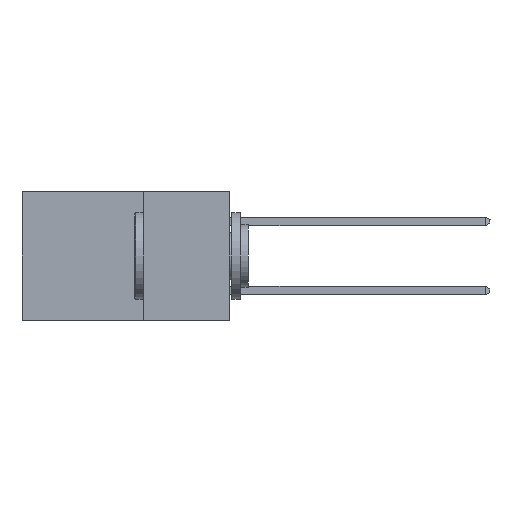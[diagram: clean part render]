
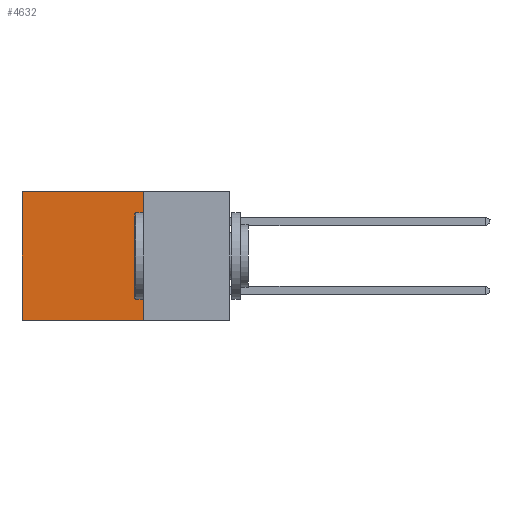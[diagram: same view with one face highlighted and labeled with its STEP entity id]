
A CAD part, left-side view. The second image highlights one B-rep face of the part: STEP entity #4632.
In plain terms, the highlighted planar face has unit normal (-1, 0, 0).
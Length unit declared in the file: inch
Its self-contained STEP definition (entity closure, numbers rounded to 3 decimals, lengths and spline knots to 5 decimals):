
#165 = LINE ( 'NONE', #15744, #16355 ) ;
#769 = EDGE_CURVE ( 'NONE', #20428, #2796, #25912, .T. ) ;
#1388 = DIRECTION ( 'NONE',  ( 0., 0., -1. ) ) ;
#1730 = CARTESIAN_POINT ( 'NONE',  ( 0.298, 0.25, -0.37 ) ) ;
#2405 = DIRECTION ( 'NONE',  ( 0., 1., 0. ) ) ;
#2796 = VERTEX_POINT ( 'NONE', #20936 ) ;
#2900 = VECTOR ( 'NONE', #12399, 39.37008 ) ;
#3042 = FACE_OUTER_BOUND ( 'NONE', #8528, .T. ) ;
#3528 = LINE ( 'NONE', #8315, #2900 ) ;
#4632 = ADVANCED_FACE ( 'NONE', ( #3042 ), #19591, .F. ) ;
#4899 = ORIENTED_EDGE ( 'NONE', *, *, #10779, .T. ) ;
#6405 = CARTESIAN_POINT ( 'NONE',  ( 0.298, 0.25, 0. ) ) ;
#6720 = VECTOR ( 'NONE', #2405, 39.37008 ) ;
#6806 = CARTESIAN_POINT ( 'NONE',  ( 0.298, 0.25, 0. ) ) ;
#6865 = DIRECTION ( 'NONE',  ( 1., 0., 0. ) ) ;
#7548 = DIRECTION ( 'NONE',  ( 0., 0., -1. ) ) ;
#8315 = CARTESIAN_POINT ( 'NONE',  ( 0.298, 0.25, -0.37 ) ) ;
#8528 = EDGE_LOOP ( 'NONE', ( #22389, #21306, #22111, #4899 ) ) ;
#10779 = EDGE_CURVE ( 'NONE', #15896, #20428, #12158, .T. ) ;
#12158 = LINE ( 'NONE', #6405, #6720 ) ;
#12399 = DIRECTION ( 'NONE',  ( 0., 1., 0. ) ) ;
#14059 = EDGE_CURVE ( 'NONE', #22234, #2796, #3528, .T. ) ;
#15744 = CARTESIAN_POINT ( 'NONE',  ( 0.298, 0.25, 0. ) ) ;
#15751 = CARTESIAN_POINT ( 'NONE',  ( 0.298, 0.6, 0. ) ) ;
#15896 = VERTEX_POINT ( 'NONE', #17859 ) ;
#16355 = VECTOR ( 'NONE', #7548, 39.37008 ) ;
#17859 = CARTESIAN_POINT ( 'NONE',  ( 0.298, 0.25, 0. ) ) ;
#19074 = EDGE_CURVE ( 'NONE', #15896, #22234, #165, .T. ) ;
#19461 = VECTOR ( 'NONE', #1388, 39.37008 ) ;
#19591 = PLANE ( 'NONE',  #25476 ) ;
#19594 = DIRECTION ( 'NONE',  ( 0., 0., -1. ) ) ;
#20428 = VERTEX_POINT ( 'NONE', #21833 ) ;
#20936 = CARTESIAN_POINT ( 'NONE',  ( 0.298, 0.6, -0.37 ) ) ;
#21306 = ORIENTED_EDGE ( 'NONE', *, *, #14059, .F. ) ;
#21833 = CARTESIAN_POINT ( 'NONE',  ( 0.298, 0.6, 0. ) ) ;
#22111 = ORIENTED_EDGE ( 'NONE', *, *, #19074, .F. ) ;
#22234 = VERTEX_POINT ( 'NONE', #1730 ) ;
#22389 = ORIENTED_EDGE ( 'NONE', *, *, #769, .T. ) ;
#25476 = AXIS2_PLACEMENT_3D ( 'NONE', #6806, #6865, #19594 ) ;
#25912 = LINE ( 'NONE', #15751, #19461 ) ;
